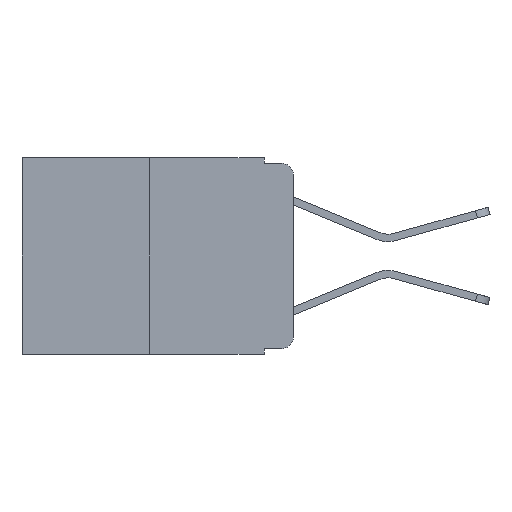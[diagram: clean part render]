
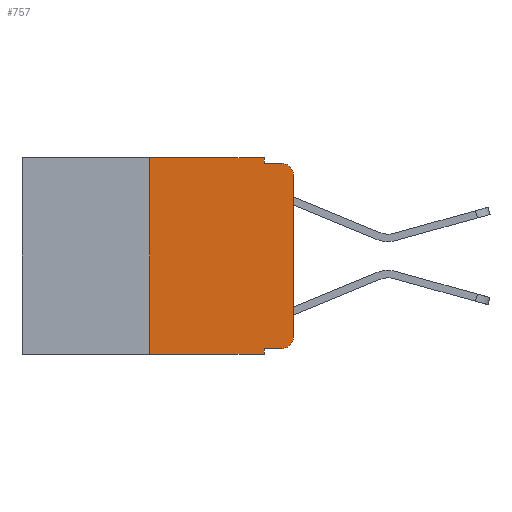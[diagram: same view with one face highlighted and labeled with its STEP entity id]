
A CAD part, left-side view. The second image highlights one B-rep face of the part: STEP entity #757.
In plain terms, the highlighted planar face has unit normal (-1, 0, 0).
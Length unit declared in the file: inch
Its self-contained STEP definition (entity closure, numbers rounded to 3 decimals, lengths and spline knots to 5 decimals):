
#220 = CARTESIAN_POINT ( 'NONE',  ( 0., 0.051, 0. ) ) ;
#450 = ORIENTED_EDGE ( 'NONE', *, *, #4243, .F. ) ;
#757 = ADVANCED_FACE ( 'NONE', ( #982 ), #14214, .F. ) ;
#982 = FACE_OUTER_BOUND ( 'NONE', #15243, .T. ) ;
#1041 = ORIENTED_EDGE ( 'NONE', *, *, #21389, .F. ) ;
#1182 = VECTOR ( 'NONE', #7313, 39.37008 ) ;
#1639 = LINE ( 'NONE', #17731, #20230 ) ;
#1739 = CIRCLE ( 'NONE', #9585, 0.02 ) ;
#1955 = CARTESIAN_POINT ( 'NONE',  ( 0., 0.051, -0.333 ) ) ;
#2277 = CARTESIAN_POINT ( 'NONE',  ( 0., 0.051, -0.01 ) ) ;
#2551 = ORIENTED_EDGE ( 'NONE', *, *, #15767, .T. ) ;
#2571 = CARTESIAN_POINT ( 'NONE',  ( 0., 0.25, 0. ) ) ;
#2652 = CARTESIAN_POINT ( 'NONE',  ( 0., 0., 0. ) ) ;
#2760 = CARTESIAN_POINT ( 'NONE',  ( 0., 0.473, 0. ) ) ;
#3437 = CARTESIAN_POINT ( 'NONE',  ( 0., 0.051, -0.333 ) ) ;
#4243 = EDGE_CURVE ( 'NONE', #19153, #10317, #5275, .T. ) ;
#4493 = DIRECTION ( 'NONE',  ( -1., 0., 0. ) ) ;
#5016 = AXIS2_PLACEMENT_3D ( 'NONE', #16441, #15885, #14015 ) ;
#5275 = LINE ( 'NONE', #15278, #13669 ) ;
#5759 = CARTESIAN_POINT ( 'NONE',  ( 0., 0.25, -0.343 ) ) ;
#6020 = LINE ( 'NONE', #2760, #19071 ) ;
#6706 = EDGE_CURVE ( 'NONE', #10317, #19301, #21580, .T. ) ;
#7003 = LINE ( 'NONE', #2571, #16418 ) ;
#7313 = DIRECTION ( 'NONE',  ( 0., -1., 0. ) ) ;
#7592 = CARTESIAN_POINT ( 'NONE',  ( 0., 0.25, 0. ) ) ;
#7735 = VERTEX_POINT ( 'NONE', #10585 ) ;
#8083 = CARTESIAN_POINT ( 'NONE',  ( 0., 0.051, -0.01 ) ) ;
#8151 = DIRECTION ( 'NONE',  ( 0., 0., 1. ) ) ;
#8783 = CARTESIAN_POINT ( 'NONE',  ( 0., 0.02, -0.313 ) ) ;
#9549 = EDGE_CURVE ( 'NONE', #19110, #7735, #19790, .T. ) ;
#9585 = AXIS2_PLACEMENT_3D ( 'NONE', #15185, #4493, #16973 ) ;
#10012 = VERTEX_POINT ( 'NONE', #3437 ) ;
#10317 = VERTEX_POINT ( 'NONE', #8083 ) ;
#10334 = EDGE_CURVE ( 'NONE', #12563, #19301, #1739, .T. ) ;
#10467 = CARTESIAN_POINT ( 'NONE',  ( 0., 0.02, -0.333 ) ) ;
#10499 = LINE ( 'NONE', #1955, #16820 ) ;
#10585 = CARTESIAN_POINT ( 'NONE',  ( 0., 0.051, -0.343 ) ) ;
#10604 = DIRECTION ( 'NONE',  ( 0., 0., -1. ) ) ;
#10715 = CARTESIAN_POINT ( 'NONE',  ( 0., 0., -0.313 ) ) ;
#11419 = ORIENTED_EDGE ( 'NONE', *, *, #9549, .T. ) ;
#11795 = LINE ( 'NONE', #2652, #15906 ) ;
#12531 = CARTESIAN_POINT ( 'NONE',  ( 0., 0.473, -0.343 ) ) ;
#12563 = VERTEX_POINT ( 'NONE', #12603 ) ;
#12603 = CARTESIAN_POINT ( 'NONE',  ( 0., 0., -0.03 ) ) ;
#12753 = ORIENTED_EDGE ( 'NONE', *, *, #10334, .T. ) ;
#13120 = EDGE_CURVE ( 'NONE', #14728, #17864, #13580, .T. ) ;
#13399 = CARTESIAN_POINT ( 'NONE',  ( 0., 0.02, -0.01 ) ) ;
#13580 = CIRCLE ( 'NONE', #16226, 0.02 ) ;
#13669 = VECTOR ( 'NONE', #15181, 39.37008 ) ;
#14015 = DIRECTION ( 'NONE',  ( 0., 0., -1. ) ) ;
#14214 = PLANE ( 'NONE',  #5016 ) ;
#14242 = DIRECTION ( 'NONE',  ( 0., 0., -1. ) ) ;
#14304 = EDGE_CURVE ( 'NONE', #10012, #14728, #10499, .T. ) ;
#14637 = DIRECTION ( 'NONE',  ( 0., -1., 0. ) ) ;
#14728 = VERTEX_POINT ( 'NONE', #10467 ) ;
#15181 = DIRECTION ( 'NONE',  ( 0., 0., -1. ) ) ;
#15185 = CARTESIAN_POINT ( 'NONE',  ( 0., 0.02, -0.03 ) ) ;
#15243 = EDGE_LOOP ( 'NONE', ( #2551, #12753, #22628, #450, #19657, #1041, #11419, #21321, #17767, #18314 ) ) ;
#15278 = CARTESIAN_POINT ( 'NONE',  ( 0., 0.051, 0. ) ) ;
#15767 = EDGE_CURVE ( 'NONE', #17864, #12563, #11795, .T. ) ;
#15885 = DIRECTION ( 'NONE',  ( 1., 0., 0. ) ) ;
#15906 = VECTOR ( 'NONE', #20582, 39.37008 ) ;
#16226 = AXIS2_PLACEMENT_3D ( 'NONE', #8783, #21131, #10604 ) ;
#16418 = VECTOR ( 'NONE', #8151, 39.37008 ) ;
#16441 = CARTESIAN_POINT ( 'NONE',  ( 0., 0.473, 0. ) ) ;
#16679 = DIRECTION ( 'NONE',  ( 0., -1., 0. ) ) ;
#16820 = VECTOR ( 'NONE', #14637, 39.37008 ) ;
#16973 = DIRECTION ( 'NONE',  ( 0., 0., -1. ) ) ;
#17377 = VERTEX_POINT ( 'NONE', #7592 ) ;
#17731 = CARTESIAN_POINT ( 'NONE',  ( 0., 0.051, 0. ) ) ;
#17767 = ORIENTED_EDGE ( 'NONE', *, *, #14304, .T. ) ;
#17864 = VERTEX_POINT ( 'NONE', #10715 ) ;
#17867 = EDGE_CURVE ( 'NONE', #10012, #7735, #1639, .T. ) ;
#18314 = ORIENTED_EDGE ( 'NONE', *, *, #13120, .T. ) ;
#18783 = EDGE_CURVE ( 'NONE', #17377, #19153, #6020, .T. ) ;
#19071 = VECTOR ( 'NONE', #20676, 39.37008 ) ;
#19110 = VERTEX_POINT ( 'NONE', #5759 ) ;
#19153 = VERTEX_POINT ( 'NONE', #220 ) ;
#19301 = VERTEX_POINT ( 'NONE', #13399 ) ;
#19657 = ORIENTED_EDGE ( 'NONE', *, *, #18783, .F. ) ;
#19790 = LINE ( 'NONE', #12531, #1182 ) ;
#20230 = VECTOR ( 'NONE', #14242, 39.37008 ) ;
#20582 = DIRECTION ( 'NONE',  ( 0., 0., 1. ) ) ;
#20676 = DIRECTION ( 'NONE',  ( 0., -1., 0. ) ) ;
#21131 = DIRECTION ( 'NONE',  ( -1., 0., 0. ) ) ;
#21321 = ORIENTED_EDGE ( 'NONE', *, *, #17867, .F. ) ;
#21389 = EDGE_CURVE ( 'NONE', #19110, #17377, #7003, .T. ) ;
#21580 = LINE ( 'NONE', #2277, #22120 ) ;
#22120 = VECTOR ( 'NONE', #16679, 39.37008 ) ;
#22628 = ORIENTED_EDGE ( 'NONE', *, *, #6706, .F. ) ;
